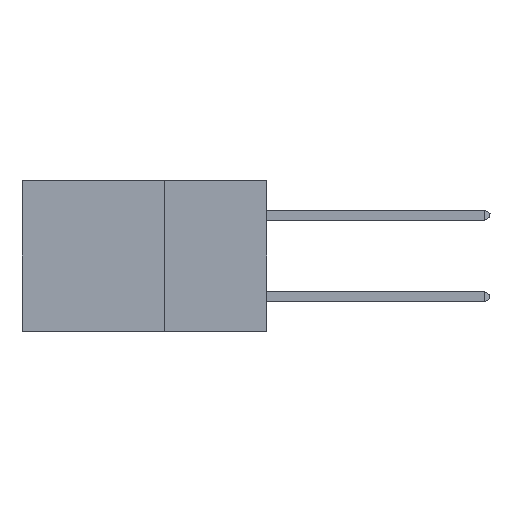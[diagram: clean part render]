
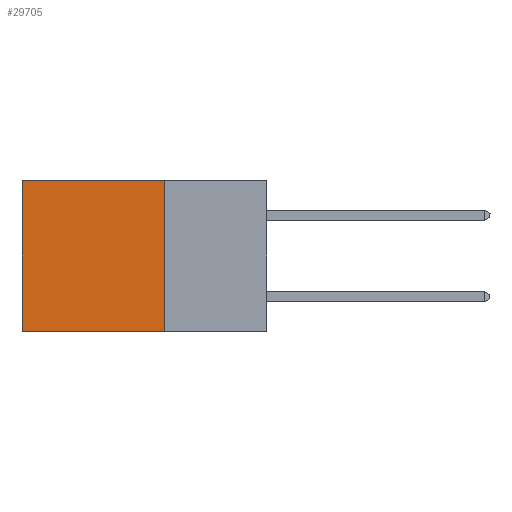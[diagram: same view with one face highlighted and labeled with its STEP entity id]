
A CAD part, left-side view. The second image highlights one B-rep face of the part: STEP entity #29705.
In plain terms, the highlighted planar face has unit normal (-1, 0, 0).
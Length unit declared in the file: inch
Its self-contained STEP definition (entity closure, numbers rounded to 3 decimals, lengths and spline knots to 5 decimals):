
#327 = DIRECTION ( 'NONE',  ( 0., 0., -1. ) ) ;
#1468 = DIRECTION ( 'NONE',  ( 0., 1., 0. ) ) ;
#2060 = ORIENTED_EDGE ( 'NONE', *, *, #21811, .T. ) ;
#2834 = LINE ( 'NONE', #30676, #15104 ) ;
#3918 = VECTOR ( 'NONE', #327, 39.37008 ) ;
#3954 = CARTESIAN_POINT ( 'NONE',  ( 0.2875, 0.6, 0. ) ) ;
#4825 = CARTESIAN_POINT ( 'NONE',  ( 0.2875, 0.25, 0. ) ) ;
#6197 = CARTESIAN_POINT ( 'NONE',  ( 0.2875, 0.25, -0.37 ) ) ;
#6738 = EDGE_LOOP ( 'NONE', ( #7836, #22907, #30870, #2060 ) ) ;
#7836 = ORIENTED_EDGE ( 'NONE', *, *, #36263, .T. ) ;
#10730 = VERTEX_POINT ( 'NONE', #32036 ) ;
#11857 = LINE ( 'NONE', #33922, #3918 ) ;
#12199 = CARTESIAN_POINT ( 'NONE',  ( 0.2875, 0.25, 0. ) ) ;
#12378 = DIRECTION ( 'NONE',  ( 0., 0., -1. ) ) ;
#13331 = DIRECTION ( 'NONE',  ( 0., 0., -1. ) ) ;
#15104 = VECTOR ( 'NONE', #21957, 39.37008 ) ;
#15618 = EDGE_CURVE ( 'NONE', #26045, #29754, #26116, .T. ) ;
#17002 = EDGE_CURVE ( 'NONE', #29754, #10730, #24116, .T. ) ;
#17325 = AXIS2_PLACEMENT_3D ( 'NONE', #21844, #36130, #13331 ) ;
#18296 = VERTEX_POINT ( 'NONE', #3954 ) ;
#19084 = PLANE ( 'NONE',  #17325 ) ;
#21811 = EDGE_CURVE ( 'NONE', #26045, #18296, #2834, .T. ) ;
#21844 = CARTESIAN_POINT ( 'NONE',  ( 0.2875, 0.25, 0. ) ) ;
#21957 = DIRECTION ( 'NONE',  ( 0., 1., 0. ) ) ;
#22907 = ORIENTED_EDGE ( 'NONE', *, *, #17002, .F. ) ;
#23231 = VECTOR ( 'NONE', #1468, 39.37008 ) ;
#24116 = LINE ( 'NONE', #6197, #23231 ) ;
#26045 = VERTEX_POINT ( 'NONE', #4825 ) ;
#26116 = LINE ( 'NONE', #12199, #30281 ) ;
#29705 = ADVANCED_FACE ( 'NONE', ( #35580 ), #19084, .F. ) ;
#29754 = VERTEX_POINT ( 'NONE', #29826 ) ;
#29826 = CARTESIAN_POINT ( 'NONE',  ( 0.2875, 0.25, -0.37 ) ) ;
#30281 = VECTOR ( 'NONE', #12378, 39.37008 ) ;
#30676 = CARTESIAN_POINT ( 'NONE',  ( 0.2875, 0.25, 0. ) ) ;
#30870 = ORIENTED_EDGE ( 'NONE', *, *, #15618, .F. ) ;
#32036 = CARTESIAN_POINT ( 'NONE',  ( 0.2875, 0.6, -0.37 ) ) ;
#33922 = CARTESIAN_POINT ( 'NONE',  ( 0.2875, 0.6, 0. ) ) ;
#35580 = FACE_OUTER_BOUND ( 'NONE', #6738, .T. ) ;
#36130 = DIRECTION ( 'NONE',  ( 1., 0., 0. ) ) ;
#36263 = EDGE_CURVE ( 'NONE', #18296, #10730, #11857, .T. ) ;
